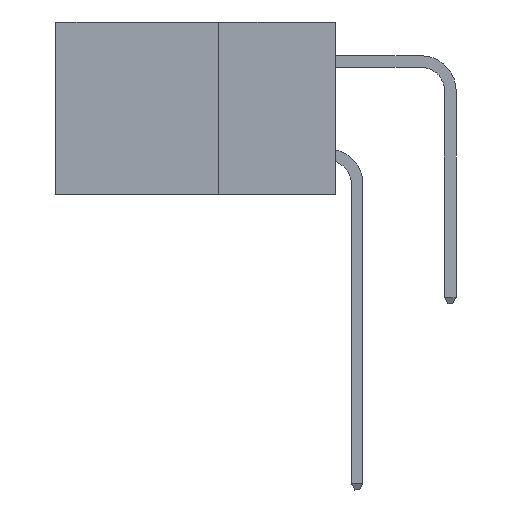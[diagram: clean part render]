
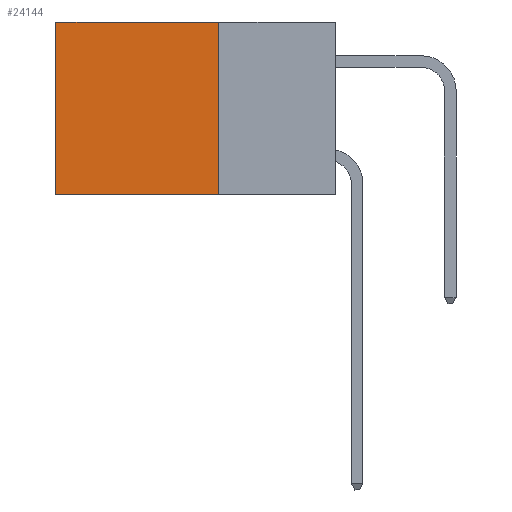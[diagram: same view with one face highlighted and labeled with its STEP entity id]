
A CAD part, left-side view. The second image highlights one B-rep face of the part: STEP entity #24144.
In plain terms, the highlighted planar face has unit normal (-1, 0, 0).
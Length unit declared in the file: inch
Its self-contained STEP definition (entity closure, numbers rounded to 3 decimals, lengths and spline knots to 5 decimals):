
#478 = CARTESIAN_POINT ( 'NONE',  ( 0.2875, 0.25, 0. ) ) ;
#602 = LINE ( 'NONE', #19609, #22845 ) ;
#690 = EDGE_LOOP ( 'NONE', ( #20227, #24421, #6680, #20003 ) ) ;
#732 = DIRECTION ( 'NONE',  ( 1., 0., 0. ) ) ;
#762 = AXIS2_PLACEMENT_3D ( 'NONE', #22562, #732, #6564 ) ;
#1920 = LINE ( 'NONE', #12339, #23217 ) ;
#5750 = EDGE_CURVE ( 'NONE', #9342, #6598, #1920, .T. ) ;
#6564 = DIRECTION ( 'NONE',  ( 0., 0., -1. ) ) ;
#6598 = VERTEX_POINT ( 'NONE', #21451 ) ;
#6680 = ORIENTED_EDGE ( 'NONE', *, *, #9440, .F. ) ;
#6737 = DIRECTION ( 'NONE',  ( 0., 1., 0. ) ) ;
#6955 = LINE ( 'NONE', #478, #16182 ) ;
#8455 = CARTESIAN_POINT ( 'NONE',  ( 0.2875, 0.6, 0. ) ) ;
#9342 = VERTEX_POINT ( 'NONE', #11609 ) ;
#9440 = EDGE_CURVE ( 'NONE', #20739, #9342, #6955, .T. ) ;
#11443 = VECTOR ( 'NONE', #24244, 39.37008 ) ;
#11609 = CARTESIAN_POINT ( 'NONE',  ( 0.2875, 0.25, -0.37 ) ) ;
#11806 = CARTESIAN_POINT ( 'NONE',  ( 0.2875, 0.6, 0. ) ) ;
#11930 = FACE_OUTER_BOUND ( 'NONE', #690, .T. ) ;
#12107 = CARTESIAN_POINT ( 'NONE',  ( 0.2875, 0.25, 0. ) ) ;
#12110 = DIRECTION ( 'NONE',  ( 0., 0., -1. ) ) ;
#12339 = CARTESIAN_POINT ( 'NONE',  ( 0.2875, 0.25, -0.37 ) ) ;
#15691 = EDGE_CURVE ( 'NONE', #20954, #6598, #23792, .T. ) ;
#16182 = VECTOR ( 'NONE', #12110, 39.37008 ) ;
#18647 = PLANE ( 'NONE',  #762 ) ;
#19379 = EDGE_CURVE ( 'NONE', #20739, #20954, #602, .T. ) ;
#19532 = DIRECTION ( 'NONE',  ( 0., 1., 0. ) ) ;
#19609 = CARTESIAN_POINT ( 'NONE',  ( 0.2875, 0.25, 0. ) ) ;
#20003 = ORIENTED_EDGE ( 'NONE', *, *, #19379, .T. ) ;
#20227 = ORIENTED_EDGE ( 'NONE', *, *, #15691, .T. ) ;
#20739 = VERTEX_POINT ( 'NONE', #12107 ) ;
#20954 = VERTEX_POINT ( 'NONE', #11806 ) ;
#21451 = CARTESIAN_POINT ( 'NONE',  ( 0.2875, 0.6, -0.37 ) ) ;
#22562 = CARTESIAN_POINT ( 'NONE',  ( 0.2875, 0.25, 0. ) ) ;
#22845 = VECTOR ( 'NONE', #19532, 39.37008 ) ;
#23217 = VECTOR ( 'NONE', #6737, 39.37008 ) ;
#23792 = LINE ( 'NONE', #8455, #11443 ) ;
#24144 = ADVANCED_FACE ( 'NONE', ( #11930 ), #18647, .F. ) ;
#24244 = DIRECTION ( 'NONE',  ( 0., 0., -1. ) ) ;
#24421 = ORIENTED_EDGE ( 'NONE', *, *, #5750, .F. ) ;
